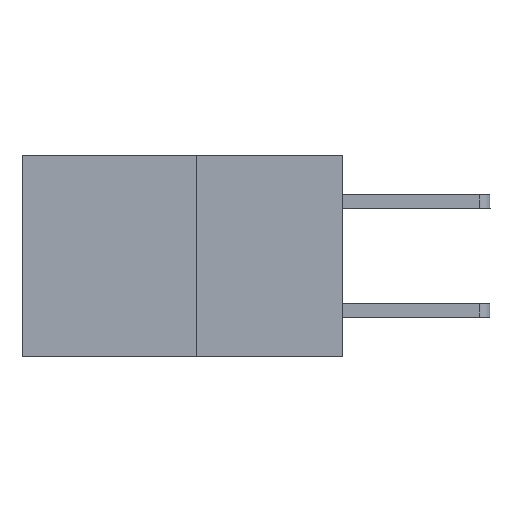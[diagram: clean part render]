
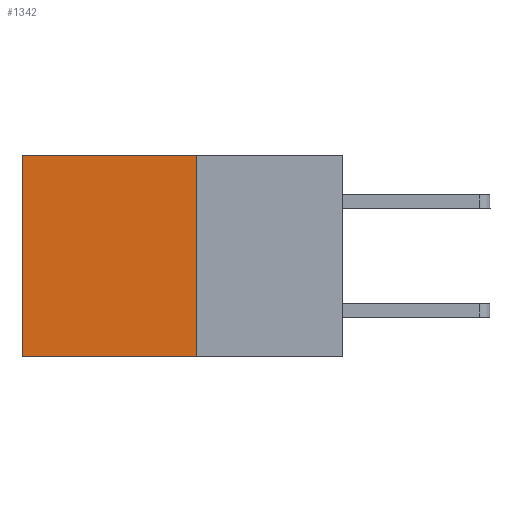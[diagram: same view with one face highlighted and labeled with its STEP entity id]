
A CAD part, left-side view. The second image highlights one B-rep face of the part: STEP entity #1342.
In plain terms, the highlighted planar face has unit normal (-1, 0, 0).
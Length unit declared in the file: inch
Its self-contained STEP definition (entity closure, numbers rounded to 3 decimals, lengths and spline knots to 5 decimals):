
#774 = LINE ( 'NONE', #2323, #2180 ) ;
#973 = VERTEX_POINT ( 'NONE', #4547 ) ;
#1065 = VECTOR ( 'NONE', #2186, 39.37008 ) ;
#1285 = LINE ( 'NONE', #2210, #1065 ) ;
#1342 = ADVANCED_FACE ( 'NONE', ( #6129 ), #5941, .F. ) ;
#1758 = CARTESIAN_POINT ( 'NONE',  ( 0.277, 0.59, 0. ) ) ;
#2134 = DIRECTION ( 'NONE',  ( 0., 0., -1. ) ) ;
#2180 = VECTOR ( 'NONE', #2389, 39.37008 ) ;
#2186 = DIRECTION ( 'NONE',  ( 0., 0., -1. ) ) ;
#2210 = CARTESIAN_POINT ( 'NONE',  ( 0.277, 0.59, -0.37 ) ) ;
#2323 = CARTESIAN_POINT ( 'NONE',  ( 0.277, 0.27, 0. ) ) ;
#2389 = DIRECTION ( 'NONE',  ( 0., 1., 0. ) ) ;
#2531 = ORIENTED_EDGE ( 'NONE', *, *, #5135, .F. ) ;
#2575 = EDGE_CURVE ( 'NONE', #4764, #5864, #7018, .T. ) ;
#3471 = EDGE_LOOP ( 'NONE', ( #5115, #5374, #2531, #6414 ) ) ;
#4102 = CARTESIAN_POINT ( 'NONE',  ( 0.277, 0.27, -0.37 ) ) ;
#4121 = CARTESIAN_POINT ( 'NONE',  ( 0.277, 0.59, -0.37 ) ) ;
#4337 = AXIS2_PLACEMENT_3D ( 'NONE', #7518, #8453, #2134 ) ;
#4547 = CARTESIAN_POINT ( 'NONE',  ( 0.277, 0.27, 0. ) ) ;
#4612 = DIRECTION ( 'NONE',  ( 0., 0., -1. ) ) ;
#4750 = LINE ( 'NONE', #4102, #8170 ) ;
#4764 = VERTEX_POINT ( 'NONE', #4944 ) ;
#4944 = CARTESIAN_POINT ( 'NONE',  ( 0.277, 0.27, -0.37 ) ) ;
#5075 = CARTESIAN_POINT ( 'NONE',  ( 0.277, 0.27, -0.37 ) ) ;
#5115 = ORIENTED_EDGE ( 'NONE', *, *, #7812, .T. ) ;
#5135 = EDGE_CURVE ( 'NONE', #973, #4764, #4750, .T. ) ;
#5351 = VECTOR ( 'NONE', #5434, 39.37008 ) ;
#5374 = ORIENTED_EDGE ( 'NONE', *, *, #2575, .F. ) ;
#5434 = DIRECTION ( 'NONE',  ( 0., 1., 0. ) ) ;
#5864 = VERTEX_POINT ( 'NONE', #4121 ) ;
#5941 = PLANE ( 'NONE',  #4337 ) ;
#6129 = FACE_OUTER_BOUND ( 'NONE', #3471, .T. ) ;
#6253 = EDGE_CURVE ( 'NONE', #973, #6648, #774, .T. ) ;
#6414 = ORIENTED_EDGE ( 'NONE', *, *, #6253, .T. ) ;
#6648 = VERTEX_POINT ( 'NONE', #1758 ) ;
#7018 = LINE ( 'NONE', #5075, #5351 ) ;
#7518 = CARTESIAN_POINT ( 'NONE',  ( 0.277, 0.27, -0.37 ) ) ;
#7812 = EDGE_CURVE ( 'NONE', #6648, #5864, #1285, .T. ) ;
#8170 = VECTOR ( 'NONE', #4612, 39.37008 ) ;
#8453 = DIRECTION ( 'NONE',  ( 1., 0., 0. ) ) ;
